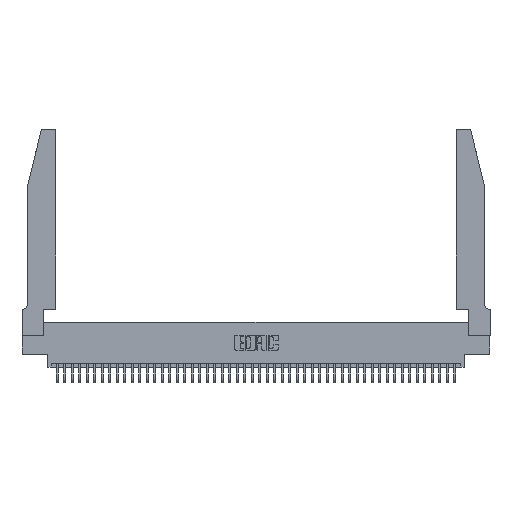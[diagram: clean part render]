
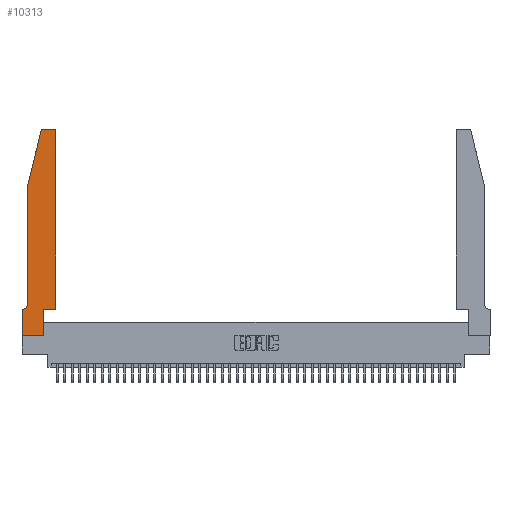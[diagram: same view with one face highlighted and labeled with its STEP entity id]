
A CAD part, top view. The second image highlights one B-rep face of the part: STEP entity #10313.
In plain terms, the highlighted planar face has unit normal (0, 0, 1).
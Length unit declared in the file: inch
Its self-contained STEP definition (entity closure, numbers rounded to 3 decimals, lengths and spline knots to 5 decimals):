
#15 = CIRCLE ( 'NONE', #27878, 0.07 ) ;
#486 = CARTESIAN_POINT ( 'NONE',  ( 0., 0., 0.37 ) ) ;
#879 = ORIENTED_EDGE ( 'NONE', *, *, #1887, .T. ) ;
#1271 = CARTESIAN_POINT ( 'NONE',  ( 0., 0., 0.37 ) ) ;
#1737 = DIRECTION ( 'NONE',  ( 0., 0., 1. ) ) ;
#1887 = EDGE_CURVE ( 'NONE', #24095, #13550, #14297, .T. ) ;
#2000 = LINE ( 'NONE', #1271, #16870 ) ;
#3436 = EDGE_CURVE ( 'NONE', #22785, #47238, #8497, .T. ) ;
#3676 = VERTEX_POINT ( 'NONE', #20705 ) ;
#4204 = VERTEX_POINT ( 'NONE', #45625 ) ;
#4977 = VERTEX_POINT ( 'NONE', #33585 ) ;
#5619 = VERTEX_POINT ( 'NONE', #11001 ) ;
#5644 = DIRECTION ( 'NONE',  ( 1., 0., 0. ) ) ;
#6008 = CARTESIAN_POINT ( 'NONE',  ( 0., 0., 0.37 ) ) ;
#7281 = EDGE_CURVE ( 'NONE', #5619, #12523, #24521, .T. ) ;
#8497 = CIRCLE ( 'NONE', #25291, 0.03 ) ;
#10313 = ADVANCED_FACE ( 'NONE', ( #34014 ), #11645, .T. ) ;
#11001 = CARTESIAN_POINT ( 'NONE',  ( 0.0755, 2., 0.37 ) ) ;
#11592 = CARTESIAN_POINT ( 'NONE',  ( 0.0755, 0.42, 0.37 ) ) ;
#11645 = PLANE ( 'NONE',  #27352 ) ;
#11900 = DIRECTION ( 'NONE',  ( -0.239, -0.971, 0. ) ) ;
#12523 = VERTEX_POINT ( 'NONE', #11592 ) ;
#12931 = DIRECTION ( 'NONE',  ( 1., 0., 0. ) ) ;
#13550 = VERTEX_POINT ( 'NONE', #15334 ) ;
#14059 = VECTOR ( 'NONE', #11900, 39.37008 ) ;
#14162 = VECTOR ( 'NONE', #19160, 39.37008 ) ;
#14297 = CIRCLE ( 'NONE', #30537, 0.03 ) ;
#14806 = VECTOR ( 'NONE', #29890, 39.37008 ) ;
#14880 = DIRECTION ( 'NONE',  ( -1., 0., 0. ) ) ;
#15334 = CARTESIAN_POINT ( 'NONE',  ( 0.25487, 2.72718, 0.37 ) ) ;
#15817 = DIRECTION ( 'NONE',  ( 1., 0., 0. ) ) ;
#15962 = DIRECTION ( 'NONE',  ( 0., 1., 0. ) ) ;
#16258 = LINE ( 'NONE', #25633, #29949 ) ;
#16870 = VECTOR ( 'NONE', #34207, 39.37008 ) ;
#16899 = CARTESIAN_POINT ( 'NONE',  ( 0.0755, 0.35, 0.37 ) ) ;
#18632 = CARTESIAN_POINT ( 'NONE',  ( 0.0755, 2., 0.37 ) ) ;
#19160 = DIRECTION ( 'NONE',  ( 0., -1., 0. ) ) ;
#19305 = ORIENTED_EDGE ( 'NONE', *, *, #38217, .T. ) ;
#19478 = EDGE_CURVE ( 'NONE', #26919, #23461, #30798, .T. ) ;
#19989 = EDGE_CURVE ( 'NONE', #4204, #45734, #34305, .T. ) ;
#20098 = VECTOR ( 'NONE', #41773, 39.37008 ) ;
#20285 = DIRECTION ( 'NONE',  ( -1., 0., 0. ) ) ;
#20541 = CARTESIAN_POINT ( 'NONE',  ( 0.4505, 0.35, 0.37 ) ) ;
#20691 = LINE ( 'NONE', #27584, #30473 ) ;
#20705 = CARTESIAN_POINT ( 'NONE',  ( 0.0055, 0.35, 0.37 ) ) ;
#20895 = CARTESIAN_POINT ( 'NONE',  ( 0.4205, 2.75, 0.37 ) ) ;
#20897 = LINE ( 'NONE', #16899, #38078 ) ;
#21060 = VECTOR ( 'NONE', #36289, 39.37008 ) ;
#21306 = EDGE_CURVE ( 'NONE', #13550, #5619, #23838, .T. ) ;
#21886 = ORIENTED_EDGE ( 'NONE', *, *, #27346, .T. ) ;
#22156 = CARTESIAN_POINT ( 'NONE',  ( 0.2865, 0.35, 0.37 ) ) ;
#22248 = ORIENTED_EDGE ( 'NONE', *, *, #45113, .T. ) ;
#22785 = VERTEX_POINT ( 'NONE', #41458 ) ;
#23461 = VERTEX_POINT ( 'NONE', #28134 ) ;
#23495 = DIRECTION ( 'NONE',  ( 0., 0., 1. ) ) ;
#23838 = LINE ( 'NONE', #18632, #14059 ) ;
#24095 = VERTEX_POINT ( 'NONE', #25188 ) ;
#24156 = ORIENTED_EDGE ( 'NONE', *, *, #3436, .T. ) ;
#24521 = LINE ( 'NONE', #26310, #14162 ) ;
#25113 = EDGE_CURVE ( 'NONE', #23461, #22785, #39525, .T. ) ;
#25188 = CARTESIAN_POINT ( 'NONE',  ( 0.284, 2.75, 0.37 ) ) ;
#25229 = ORIENTED_EDGE ( 'NONE', *, *, #25113, .T. ) ;
#25291 = AXIS2_PLACEMENT_3D ( 'NONE', #41861, #1737, #12931 ) ;
#25633 = CARTESIAN_POINT ( 'NONE',  ( 0.2605, 2.75, 0.37 ) ) ;
#26310 = CARTESIAN_POINT ( 'NONE',  ( 0.0755, 2., 0.37 ) ) ;
#26919 = VERTEX_POINT ( 'NONE', #22156 ) ;
#27099 = ORIENTED_EDGE ( 'NONE', *, *, #19989, .T. ) ;
#27346 = EDGE_CURVE ( 'NONE', #12523, #3676, #15, .T. ) ;
#27352 = AXIS2_PLACEMENT_3D ( 'NONE', #45342, #23495, #15817 ) ;
#27584 = CARTESIAN_POINT ( 'NONE',  ( 0.2865, 0.35, 0.37 ) ) ;
#27878 = AXIS2_PLACEMENT_3D ( 'NONE', #32953, #29437, #14880 ) ;
#28134 = CARTESIAN_POINT ( 'NONE',  ( 0.4505, 0.35, 0.37 ) ) ;
#29058 = CARTESIAN_POINT ( 'NONE',  ( 0.4505, 0.35, 0.37 ) ) ;
#29437 = DIRECTION ( 'NONE',  ( 0., 0., -1. ) ) ;
#29890 = DIRECTION ( 'NONE',  ( 0., -1., 0. ) ) ;
#29949 = VECTOR ( 'NONE', #36901, 39.37008 ) ;
#30473 = VECTOR ( 'NONE', #15962, 39.37008 ) ;
#30537 = AXIS2_PLACEMENT_3D ( 'NONE', #41757, #42068, #5644 ) ;
#30798 = LINE ( 'NONE', #29058, #21060 ) ;
#32245 = ORIENTED_EDGE ( 'NONE', *, *, #19478, .T. ) ;
#32372 = ORIENTED_EDGE ( 'NONE', *, *, #33296, .T. ) ;
#32953 = CARTESIAN_POINT ( 'NONE',  ( 0.0055, 0.42, 0.37 ) ) ;
#33296 = EDGE_CURVE ( 'NONE', #47238, #24095, #16258, .T. ) ;
#33585 = CARTESIAN_POINT ( 'NONE',  ( 0.2865, 0., 0.37 ) ) ;
#34014 = FACE_OUTER_BOUND ( 'NONE', #42025, .T. ) ;
#34207 = DIRECTION ( 'NONE',  ( 1., 0., 0. ) ) ;
#34305 = LINE ( 'NONE', #486, #14806 ) ;
#36289 = DIRECTION ( 'NONE',  ( 1., 0., 0. ) ) ;
#36901 = DIRECTION ( 'NONE',  ( -1., 0., 0. ) ) ;
#38078 = VECTOR ( 'NONE', #20285, 39.37008 ) ;
#38217 = EDGE_CURVE ( 'NONE', #3676, #4204, #20897, .T. ) ;
#39069 = ORIENTED_EDGE ( 'NONE', *, *, #46737, .T. ) ;
#39172 = ORIENTED_EDGE ( 'NONE', *, *, #21306, .T. ) ;
#39525 = LINE ( 'NONE', #20541, #20098 ) ;
#41458 = CARTESIAN_POINT ( 'NONE',  ( 0.4505, 2.72, 0.37 ) ) ;
#41757 = CARTESIAN_POINT ( 'NONE',  ( 0.284, 2.72, 0.37 ) ) ;
#41773 = DIRECTION ( 'NONE',  ( 0., 1., 0. ) ) ;
#41861 = CARTESIAN_POINT ( 'NONE',  ( 0.4205, 2.72, 0.37 ) ) ;
#42025 = EDGE_LOOP ( 'NONE', ( #32372, #879, #39172, #43437, #21886, #19305, #27099, #39069, #22248, #32245, #25229, #24156 ) ) ;
#42068 = DIRECTION ( 'NONE',  ( 0., 0., 1. ) ) ;
#43437 = ORIENTED_EDGE ( 'NONE', *, *, #7281, .T. ) ;
#45113 = EDGE_CURVE ( 'NONE', #4977, #26919, #20691, .T. ) ;
#45342 = CARTESIAN_POINT ( 'NONE',  ( 0., 0.35, 0.37 ) ) ;
#45625 = CARTESIAN_POINT ( 'NONE',  ( 0., 0.35, 0.37 ) ) ;
#45734 = VERTEX_POINT ( 'NONE', #6008 ) ;
#46737 = EDGE_CURVE ( 'NONE', #45734, #4977, #2000, .T. ) ;
#47238 = VERTEX_POINT ( 'NONE', #20895 ) ;
